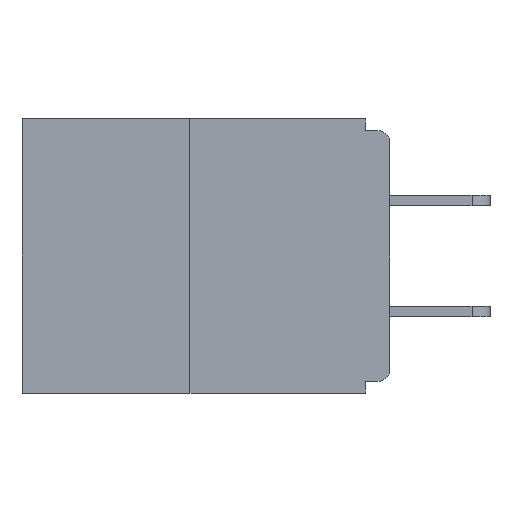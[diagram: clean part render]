
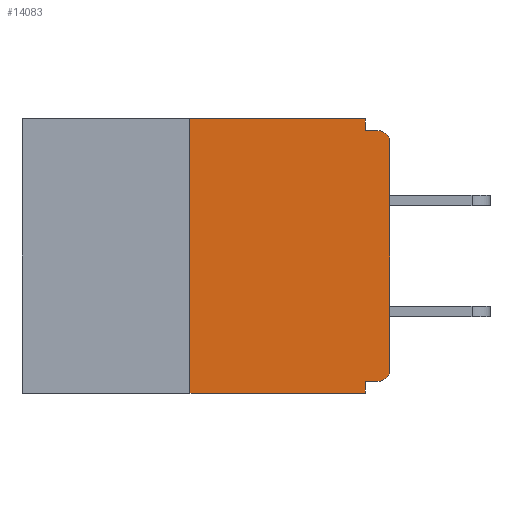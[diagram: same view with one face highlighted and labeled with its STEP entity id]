
A CAD part, left-side view. The second image highlights one B-rep face of the part: STEP entity #14083.
In plain terms, the highlighted planar face has unit normal (-1, 0, 0).
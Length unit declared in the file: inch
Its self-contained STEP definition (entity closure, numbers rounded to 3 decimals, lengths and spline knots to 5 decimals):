
#74 = VERTEX_POINT ( 'NONE', #2972 ) ;
#369 = DIRECTION ( 'NONE',  ( 0., -1., 0. ) ) ;
#386 = LINE ( 'NONE', #439, #11954 ) ;
#439 = CARTESIAN_POINT ( 'NONE',  ( 0., 0.46, -0.343 ) ) ;
#1011 = VERTEX_POINT ( 'NONE', #10165 ) ;
#1139 = CARTESIAN_POINT ( 'NONE',  ( 0., 0.031, 0. ) ) ;
#1237 = VERTEX_POINT ( 'NONE', #1139 ) ;
#1393 = VERTEX_POINT ( 'NONE', #9049 ) ;
#1413 = DIRECTION ( 'NONE',  ( -1., 0., 0. ) ) ;
#2377 = DIRECTION ( 'NONE',  ( 1., 0., 0. ) ) ;
#2435 = CARTESIAN_POINT ( 'NONE',  ( 0., 0.015, -0.328 ) ) ;
#2515 = CARTESIAN_POINT ( 'NONE',  ( 0., 0.46, 0. ) ) ;
#2972 = CARTESIAN_POINT ( 'NONE',  ( 0., 0.25, -0.343 ) ) ;
#3008 = CARTESIAN_POINT ( 'NONE',  ( 0., 0.031, -0.343 ) ) ;
#3359 = ORIENTED_EDGE ( 'NONE', *, *, #14996, .T. ) ;
#3482 = LINE ( 'NONE', #17814, #15502 ) ;
#3630 = VECTOR ( 'NONE', #15210, 39.37008 ) ;
#3900 = DIRECTION ( 'NONE',  ( 0., 0., -1. ) ) ;
#4039 = LINE ( 'NONE', #3008, #18717 ) ;
#4604 = ORIENTED_EDGE ( 'NONE', *, *, #16126, .F. ) ;
#4926 = VERTEX_POINT ( 'NONE', #15046 ) ;
#5096 = VECTOR ( 'NONE', #9438, 39.37008 ) ;
#5157 = ORIENTED_EDGE ( 'NONE', *, *, #17485, .F. ) ;
#5742 = DIRECTION ( 'NONE',  ( 0., 0., 1. ) ) ;
#5956 = DIRECTION ( 'NONE',  ( 0., 0., 1. ) ) ;
#6240 = VECTOR ( 'NONE', #10650, 39.37008 ) ;
#6314 = DIRECTION ( 'NONE',  ( -1., 0., 0. ) ) ;
#6492 = CARTESIAN_POINT ( 'NONE',  ( 0., 0.46, 0. ) ) ;
#6991 = VERTEX_POINT ( 'NONE', #15377 ) ;
#7040 = PLANE ( 'NONE',  #10148 ) ;
#7490 = CARTESIAN_POINT ( 'NONE',  ( 0., 0., -0.015 ) ) ;
#7521 = DIRECTION ( 'NONE',  ( 0., 0., -1. ) ) ;
#7647 = EDGE_CURVE ( 'NONE', #74, #4926, #3482, .T. ) ;
#7660 = ORIENTED_EDGE ( 'NONE', *, *, #15259, .T. ) ;
#8229 = EDGE_CURVE ( 'NONE', #1011, #15723, #9315, .T. ) ;
#8284 = ORIENTED_EDGE ( 'NONE', *, *, #11850, .T. ) ;
#8758 = EDGE_CURVE ( 'NONE', #19291, #1393, #9768, .T. ) ;
#8911 = DIRECTION ( 'NONE',  ( 0., 0., -1. ) ) ;
#8919 = ORIENTED_EDGE ( 'NONE', *, *, #8229, .T. ) ;
#8929 = ORIENTED_EDGE ( 'NONE', *, *, #8758, .F. ) ;
#8969 = CARTESIAN_POINT ( 'NONE',  ( 0., 0., -0.03 ) ) ;
#9049 = CARTESIAN_POINT ( 'NONE',  ( 0., 0.015, -0.015 ) ) ;
#9314 = LINE ( 'NONE', #6492, #5096 ) ;
#9315 = LINE ( 'NONE', #9758, #16208 ) ;
#9382 = AXIS2_PLACEMENT_3D ( 'NONE', #17991, #1413, #8911 ) ;
#9399 = CARTESIAN_POINT ( 'NONE',  ( 0., 0.015, -0.313 ) ) ;
#9438 = DIRECTION ( 'NONE',  ( 0., -1., 0. ) ) ;
#9467 = DIRECTION ( 'NONE',  ( 0., 0., -1. ) ) ;
#9758 = CARTESIAN_POINT ( 'NONE',  ( 0., 0., 0. ) ) ;
#9768 = LINE ( 'NONE', #7490, #6240 ) ;
#10148 = AXIS2_PLACEMENT_3D ( 'NONE', #2515, #2377, #3900 ) ;
#10165 = CARTESIAN_POINT ( 'NONE',  ( 0., 0., -0.313 ) ) ;
#10483 = CARTESIAN_POINT ( 'NONE',  ( 0., 0.031, 0. ) ) ;
#10609 = LINE ( 'NONE', #10483, #18215 ) ;
#10650 = DIRECTION ( 'NONE',  ( 0., -1., 0. ) ) ;
#11573 = EDGE_LOOP ( 'NONE', ( #4604, #17805, #7660, #14145, #5157, #3359, #8919, #8284, #8929, #12939 ) ) ;
#11775 = EDGE_CURVE ( 'NONE', #1237, #19291, #10609, .T. ) ;
#11786 = CIRCLE ( 'NONE', #9382, 0.015 ) ;
#11850 = EDGE_CURVE ( 'NONE', #15723, #1393, #11786, .T. ) ;
#11954 = VECTOR ( 'NONE', #369, 39.37008 ) ;
#12312 = VERTEX_POINT ( 'NONE', #2435 ) ;
#12939 = ORIENTED_EDGE ( 'NONE', *, *, #11775, .F. ) ;
#12959 = AXIS2_PLACEMENT_3D ( 'NONE', #9399, #6314, #9467 ) ;
#13564 = DIRECTION ( 'NONE',  ( 0., 0., -1. ) ) ;
#13682 = CARTESIAN_POINT ( 'NONE',  ( 0., 0., -0.328 ) ) ;
#14083 = ADVANCED_FACE ( 'NONE', ( #17487 ), #7040, .F. ) ;
#14145 = ORIENTED_EDGE ( 'NONE', *, *, #19272, .F. ) ;
#14996 = EDGE_CURVE ( 'NONE', #12312, #1011, #18148, .T. ) ;
#15046 = CARTESIAN_POINT ( 'NONE',  ( 0., 0.25, 0. ) ) ;
#15210 = DIRECTION ( 'NONE',  ( 0., 1., 0. ) ) ;
#15259 = EDGE_CURVE ( 'NONE', #74, #6991, #386, .T. ) ;
#15377 = CARTESIAN_POINT ( 'NONE',  ( 0., 0.031, -0.343 ) ) ;
#15502 = VECTOR ( 'NONE', #5956, 39.37008 ) ;
#15723 = VERTEX_POINT ( 'NONE', #8969 ) ;
#16126 = EDGE_CURVE ( 'NONE', #4926, #1237, #9314, .T. ) ;
#16208 = VECTOR ( 'NONE', #5742, 39.37008 ) ;
#16737 = VERTEX_POINT ( 'NONE', #17886 ) ;
#17485 = EDGE_CURVE ( 'NONE', #12312, #16737, #18781, .T. ) ;
#17487 = FACE_OUTER_BOUND ( 'NONE', #11573, .T. ) ;
#17805 = ORIENTED_EDGE ( 'NONE', *, *, #7647, .F. ) ;
#17814 = CARTESIAN_POINT ( 'NONE',  ( 0., 0.25, 0. ) ) ;
#17886 = CARTESIAN_POINT ( 'NONE',  ( 0., 0.031, -0.328 ) ) ;
#17991 = CARTESIAN_POINT ( 'NONE',  ( 0., 0.015, -0.03 ) ) ;
#18148 = CIRCLE ( 'NONE', #12959, 0.015 ) ;
#18215 = VECTOR ( 'NONE', #7521, 39.37008 ) ;
#18218 = CARTESIAN_POINT ( 'NONE',  ( 0., 0.031, -0.015 ) ) ;
#18717 = VECTOR ( 'NONE', #13564, 39.37008 ) ;
#18781 = LINE ( 'NONE', #13682, #3630 ) ;
#19272 = EDGE_CURVE ( 'NONE', #16737, #6991, #4039, .T. ) ;
#19291 = VERTEX_POINT ( 'NONE', #18218 ) ;
